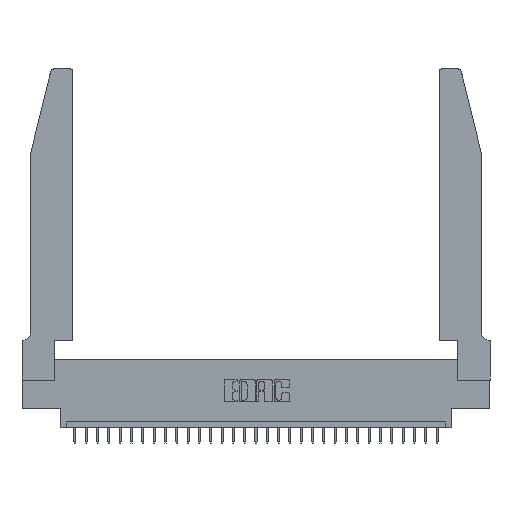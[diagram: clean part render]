
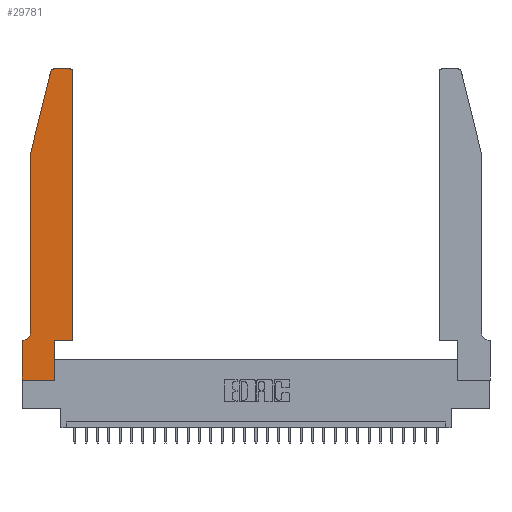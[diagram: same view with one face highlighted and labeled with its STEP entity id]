
A CAD part, top view. The second image highlights one B-rep face of the part: STEP entity #29781.
In plain terms, the highlighted planar face has unit normal (0, 0, 1).
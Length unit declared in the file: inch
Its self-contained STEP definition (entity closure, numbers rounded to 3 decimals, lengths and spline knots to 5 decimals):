
#331 = EDGE_CURVE ( 'NONE', #27604, #20199, #23206, .T. ) ;
#366 = ORIENTED_EDGE ( 'NONE', *, *, #1452, .T. ) ;
#491 = VERTEX_POINT ( 'NONE', #26195 ) ;
#934 = LINE ( 'NONE', #10484, #11266 ) ;
#1187 = FACE_OUTER_BOUND ( 'NONE', #6425, .T. ) ;
#1413 = DIRECTION ( 'NONE',  ( 0., 1., 0. ) ) ;
#1452 = EDGE_CURVE ( 'NONE', #13180, #14959, #15037, .T. ) ;
#3111 = DIRECTION ( 'NONE',  ( 0., -1., 0. ) ) ;
#3139 = CARTESIAN_POINT ( 'NONE',  ( 0.4505, 0.35, 0.37 ) ) ;
#3509 = EDGE_CURVE ( 'NONE', #14959, #22297, #11116, .T. ) ;
#3636 = CARTESIAN_POINT ( 'NONE',  ( 0.2865, 0.35, 0.37 ) ) ;
#3747 = CARTESIAN_POINT ( 'NONE',  ( 0., 0.35, 0.37 ) ) ;
#3952 = LINE ( 'NONE', #3636, #11663 ) ;
#4325 = DIRECTION ( 'NONE',  ( 0., -1., 0. ) ) ;
#5818 = DIRECTION ( 'NONE',  ( 0., 1., 0. ) ) ;
#6044 = DIRECTION ( 'NONE',  ( 1., 0., 0. ) ) ;
#6144 = VECTOR ( 'NONE', #4325, 39.37008 ) ;
#6415 = ORIENTED_EDGE ( 'NONE', *, *, #331, .T. ) ;
#6425 = EDGE_LOOP ( 'NONE', ( #8367, #23741, #16935, #366, #23598, #8128, #25439, #29149, #18468, #30917, #24503, #6415 ) ) ;
#6900 = VECTOR ( 'NONE', #12239, 39.37008 ) ;
#6906 = DIRECTION ( 'NONE',  ( 1., 0., 0. ) ) ;
#7025 = EDGE_CURVE ( 'NONE', #18969, #22900, #3952, .T. ) ;
#8128 = ORIENTED_EDGE ( 'NONE', *, *, #10510, .T. ) ;
#8209 = DIRECTION ( 'NONE',  ( 0., 0., -1. ) ) ;
#8230 = LINE ( 'NONE', #17807, #6144 ) ;
#8367 = ORIENTED_EDGE ( 'NONE', *, *, #24622, .T. ) ;
#8471 = DIRECTION ( 'NONE',  ( 1., 0., 0. ) ) ;
#8912 = EDGE_CURVE ( 'NONE', #18768, #18969, #934, .T. ) ;
#9129 = AXIS2_PLACEMENT_3D ( 'NONE', #27847, #15304, #6044 ) ;
#10357 = VECTOR ( 'NONE', #1413, 39.37008 ) ;
#10484 = CARTESIAN_POINT ( 'NONE',  ( 0., 0., 0.37 ) ) ;
#10510 = EDGE_CURVE ( 'NONE', #22297, #26915, #28878, .T. ) ;
#10586 = PLANE ( 'NONE',  #9129 ) ;
#11116 = CIRCLE ( 'NONE', #25138, 0.07 ) ;
#11266 = VECTOR ( 'NONE', #28216, 39.37008 ) ;
#11474 = CARTESIAN_POINT ( 'NONE',  ( 0.4205, 2.75, 0.37 ) ) ;
#11663 = VECTOR ( 'NONE', #5818, 39.37008 ) ;
#12239 = DIRECTION ( 'NONE',  ( -0.239, -0.971, 0. ) ) ;
#12864 = LINE ( 'NONE', #24621, #6900 ) ;
#13180 = VERTEX_POINT ( 'NONE', #18199 ) ;
#13315 = EDGE_CURVE ( 'NONE', #491, #27604, #30446, .T. ) ;
#13707 = AXIS2_PLACEMENT_3D ( 'NONE', #23526, #16174, #6906 ) ;
#13773 = EDGE_CURVE ( 'NONE', #30343, #15205, #28942, .T. ) ;
#13846 = VECTOR ( 'NONE', #16636, 39.37008 ) ;
#14133 = CARTESIAN_POINT ( 'NONE',  ( 0.0755, 0.35, 0.37 ) ) ;
#14192 = EDGE_CURVE ( 'NONE', #22900, #491, #24938, .T. ) ;
#14432 = CARTESIAN_POINT ( 'NONE',  ( 0.2865, 0., 0.37 ) ) ;
#14959 = VERTEX_POINT ( 'NONE', #15920 ) ;
#15037 = LINE ( 'NONE', #22387, #17381 ) ;
#15188 = DIRECTION ( 'NONE',  ( -1., 0., 0. ) ) ;
#15205 = VERTEX_POINT ( 'NONE', #29362 ) ;
#15304 = DIRECTION ( 'NONE',  ( 0., 0., 1. ) ) ;
#15920 = CARTESIAN_POINT ( 'NONE',  ( 0.0755, 0.42, 0.37 ) ) ;
#16174 = DIRECTION ( 'NONE',  ( 0., 0., 1. ) ) ;
#16636 = DIRECTION ( 'NONE',  ( -1., 0., 0. ) ) ;
#16935 = ORIENTED_EDGE ( 'NONE', *, *, #23006, .T. ) ;
#17060 = LINE ( 'NONE', #19552, #24507 ) ;
#17381 = VECTOR ( 'NONE', #3111, 39.37008 ) ;
#17807 = CARTESIAN_POINT ( 'NONE',  ( 0., 0., 0.37 ) ) ;
#18199 = CARTESIAN_POINT ( 'NONE',  ( 0.0755, 2., 0.37 ) ) ;
#18227 = CARTESIAN_POINT ( 'NONE',  ( 0., 0., 0.37 ) ) ;
#18468 = ORIENTED_EDGE ( 'NONE', *, *, #7025, .T. ) ;
#18691 = CARTESIAN_POINT ( 'NONE',  ( 0.284, 2.75, 0.37 ) ) ;
#18768 = VERTEX_POINT ( 'NONE', #18227 ) ;
#18969 = VERTEX_POINT ( 'NONE', #14432 ) ;
#19552 = CARTESIAN_POINT ( 'NONE',  ( 0.2605, 2.75, 0.37 ) ) ;
#20008 = CARTESIAN_POINT ( 'NONE',  ( 0.0055, 0.35, 0.37 ) ) ;
#20199 = VERTEX_POINT ( 'NONE', #11474 ) ;
#20490 = DIRECTION ( 'NONE',  ( 0., 0., 1. ) ) ;
#20688 = CARTESIAN_POINT ( 'NONE',  ( 0.4505, 0.35, 0.37 ) ) ;
#20804 = CARTESIAN_POINT ( 'NONE',  ( 0.284, 2.72, 0.37 ) ) ;
#21182 = CARTESIAN_POINT ( 'NONE',  ( 0.2865, 0.35, 0.37 ) ) ;
#22297 = VERTEX_POINT ( 'NONE', #20008 ) ;
#22387 = CARTESIAN_POINT ( 'NONE',  ( 0.0755, 2., 0.37 ) ) ;
#22900 = VERTEX_POINT ( 'NONE', #21182 ) ;
#23006 = EDGE_CURVE ( 'NONE', #15205, #13180, #12864, .T. ) ;
#23206 = CIRCLE ( 'NONE', #13707, 0.03 ) ;
#23420 = AXIS2_PLACEMENT_3D ( 'NONE', #20804, #20490, #30407 ) ;
#23526 = CARTESIAN_POINT ( 'NONE',  ( 0.4205, 2.72, 0.37 ) ) ;
#23598 = ORIENTED_EDGE ( 'NONE', *, *, #3509, .T. ) ;
#23741 = ORIENTED_EDGE ( 'NONE', *, *, #13773, .T. ) ;
#24503 = ORIENTED_EDGE ( 'NONE', *, *, #13315, .T. ) ;
#24507 = VECTOR ( 'NONE', #15188, 39.37008 ) ;
#24621 = CARTESIAN_POINT ( 'NONE',  ( 0.0755, 2., 0.37 ) ) ;
#24622 = EDGE_CURVE ( 'NONE', #20199, #30343, #17060, .T. ) ;
#24938 = LINE ( 'NONE', #3139, #28963 ) ;
#25138 = AXIS2_PLACEMENT_3D ( 'NONE', #30198, #8209, #30353 ) ;
#25439 = ORIENTED_EDGE ( 'NONE', *, *, #29835, .T. ) ;
#25613 = CARTESIAN_POINT ( 'NONE',  ( 0.4505, 2.72, 0.37 ) ) ;
#26195 = CARTESIAN_POINT ( 'NONE',  ( 0.4505, 0.35, 0.37 ) ) ;
#26915 = VERTEX_POINT ( 'NONE', #3747 ) ;
#27604 = VERTEX_POINT ( 'NONE', #25613 ) ;
#27847 = CARTESIAN_POINT ( 'NONE',  ( 0., 0.35, 0.37 ) ) ;
#28216 = DIRECTION ( 'NONE',  ( 1., 0., 0. ) ) ;
#28878 = LINE ( 'NONE', #14133, #13846 ) ;
#28942 = CIRCLE ( 'NONE', #23420, 0.03 ) ;
#28963 = VECTOR ( 'NONE', #8471, 39.37008 ) ;
#29149 = ORIENTED_EDGE ( 'NONE', *, *, #8912, .T. ) ;
#29362 = CARTESIAN_POINT ( 'NONE',  ( 0.25487, 2.72718, 0.37 ) ) ;
#29781 = ADVANCED_FACE ( 'NONE', ( #1187 ), #10586, .T. ) ;
#29835 = EDGE_CURVE ( 'NONE', #26915, #18768, #8230, .T. ) ;
#30198 = CARTESIAN_POINT ( 'NONE',  ( 0.0055, 0.42, 0.37 ) ) ;
#30343 = VERTEX_POINT ( 'NONE', #18691 ) ;
#30353 = DIRECTION ( 'NONE',  ( -1., 0., 0. ) ) ;
#30407 = DIRECTION ( 'NONE',  ( 1., 0., 0. ) ) ;
#30446 = LINE ( 'NONE', #20688, #10357 ) ;
#30917 = ORIENTED_EDGE ( 'NONE', *, *, #14192, .T. ) ;
